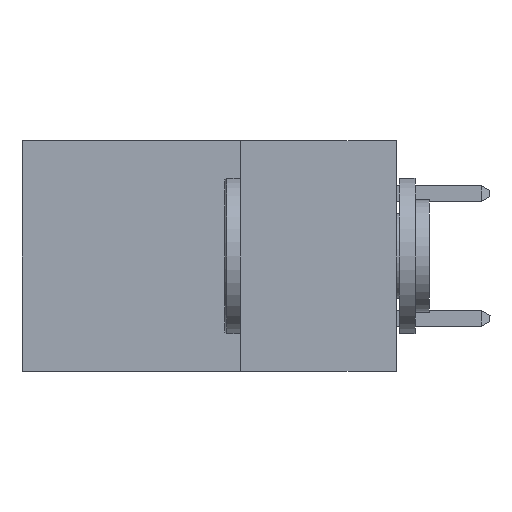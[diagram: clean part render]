
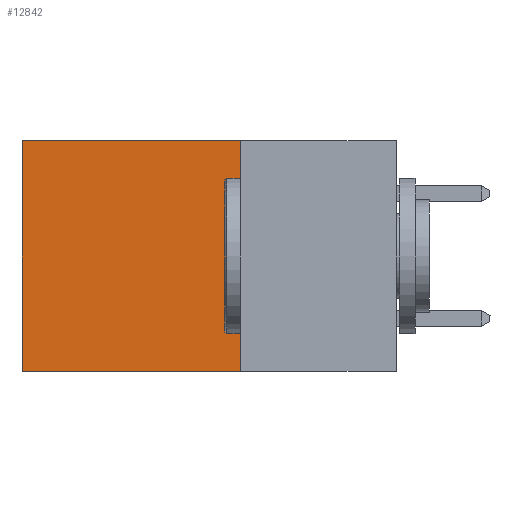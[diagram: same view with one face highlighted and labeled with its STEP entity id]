
A CAD part, left-side view. The second image highlights one B-rep face of the part: STEP entity #12842.
In plain terms, the highlighted planar face has unit normal (-1, 0, 0).
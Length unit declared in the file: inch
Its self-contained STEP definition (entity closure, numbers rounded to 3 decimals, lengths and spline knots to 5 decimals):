
#311 = DIRECTION ( 'NONE',  ( 0., 1., 0. ) ) ;
#495 = DIRECTION ( 'NONE',  ( 0., 1., 0. ) ) ;
#2255 = EDGE_CURVE ( 'NONE', #10296, #19593, #21241, .T. ) ;
#2256 = VECTOR ( 'NONE', #11616, 39.37008 ) ;
#2747 = LINE ( 'NONE', #12813, #5767 ) ;
#2988 = LINE ( 'NONE', #9017, #7683 ) ;
#3190 = ORIENTED_EDGE ( 'NONE', *, *, #19523, .F. ) ;
#4830 = EDGE_LOOP ( 'NONE', ( #7446, #3190, #14612, #8683 ) ) ;
#5111 = VERTEX_POINT ( 'NONE', #12881 ) ;
#5767 = VECTOR ( 'NONE', #495, 39.37008 ) ;
#5821 = PLANE ( 'NONE',  #12675 ) ;
#6306 = CARTESIAN_POINT ( 'NONE',  ( 0.2615, 0.25, 0. ) ) ;
#7336 = VECTOR ( 'NONE', #311, 39.37008 ) ;
#7446 = ORIENTED_EDGE ( 'NONE', *, *, #11532, .T. ) ;
#7683 = VECTOR ( 'NONE', #17687, 39.37008 ) ;
#8683 = ORIENTED_EDGE ( 'NONE', *, *, #2255, .T. ) ;
#9017 = CARTESIAN_POINT ( 'NONE',  ( 0.2615, 0.25, -0.37 ) ) ;
#9396 = DIRECTION ( 'NONE',  ( 1., 0., 0. ) ) ;
#9514 = CARTESIAN_POINT ( 'NONE',  ( 0.2615, 0.6, 0. ) ) ;
#9840 = CARTESIAN_POINT ( 'NONE',  ( 0.2615, 0.6, -0.37 ) ) ;
#10296 = VERTEX_POINT ( 'NONE', #6306 ) ;
#11532 = EDGE_CURVE ( 'NONE', #19593, #19459, #16266, .T. ) ;
#11616 = DIRECTION ( 'NONE',  ( 0., 0., -1. ) ) ;
#12675 = AXIS2_PLACEMENT_3D ( 'NONE', #18043, #9396, #21525 ) ;
#12813 = CARTESIAN_POINT ( 'NONE',  ( 0.2615, 0.25, -0.37 ) ) ;
#12842 = ADVANCED_FACE ( 'NONE', ( #21322 ), #5821, .F. ) ;
#12881 = CARTESIAN_POINT ( 'NONE',  ( 0.2615, 0.25, -0.37 ) ) ;
#14612 = ORIENTED_EDGE ( 'NONE', *, *, #20090, .F. ) ;
#16106 = CARTESIAN_POINT ( 'NONE',  ( 0.2615, 0.25, 0. ) ) ;
#16158 = CARTESIAN_POINT ( 'NONE',  ( 0.2615, 0.6, -0.37 ) ) ;
#16266 = LINE ( 'NONE', #9840, #2256 ) ;
#17687 = DIRECTION ( 'NONE',  ( 0., 0., -1. ) ) ;
#18043 = CARTESIAN_POINT ( 'NONE',  ( 0.2615, 0.25, -0.37 ) ) ;
#19459 = VERTEX_POINT ( 'NONE', #16158 ) ;
#19523 = EDGE_CURVE ( 'NONE', #5111, #19459, #2747, .T. ) ;
#19593 = VERTEX_POINT ( 'NONE', #9514 ) ;
#20090 = EDGE_CURVE ( 'NONE', #10296, #5111, #2988, .T. ) ;
#21241 = LINE ( 'NONE', #16106, #7336 ) ;
#21322 = FACE_OUTER_BOUND ( 'NONE', #4830, .T. ) ;
#21525 = DIRECTION ( 'NONE',  ( 0., 0., -1. ) ) ;
